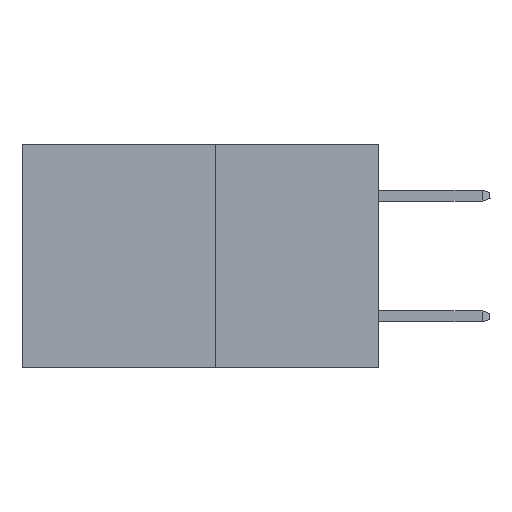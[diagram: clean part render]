
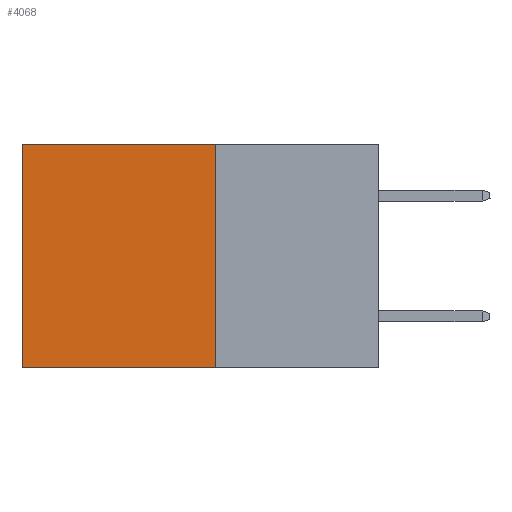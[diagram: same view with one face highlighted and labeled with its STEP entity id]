
A CAD part, left-side view. The second image highlights one B-rep face of the part: STEP entity #4068.
In plain terms, the highlighted planar face has unit normal (-1, 0, 0).
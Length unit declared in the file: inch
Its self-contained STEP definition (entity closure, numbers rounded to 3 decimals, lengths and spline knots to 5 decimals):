
#2 = EDGE_CURVE ( 'NONE', #4968, #7295, #2252, .T. ) ;
#373 = DIRECTION ( 'NONE',  ( 0., 1., 0. ) ) ;
#1313 = CARTESIAN_POINT ( 'NONE',  ( 0.277, 0.27, -0.37 ) ) ;
#2153 = CARTESIAN_POINT ( 'NONE',  ( 0.277, 0.59, -0.37 ) ) ;
#2252 = LINE ( 'NONE', #7698, #13037 ) ;
#2348 = VECTOR ( 'NONE', #8256, 39.37008 ) ;
#3199 = EDGE_CURVE ( 'NONE', #11133, #3321, #8616, .T. ) ;
#3321 = VERTEX_POINT ( 'NONE', #1313 ) ;
#3375 = AXIS2_PLACEMENT_3D ( 'NONE', #12859, #12370, #12385 ) ;
#3551 = LINE ( 'NONE', #4149, #8807 ) ;
#3883 = ORIENTED_EDGE ( 'NONE', *, *, #12152, .T. ) ;
#4068 = ADVANCED_FACE ( 'NONE', ( #10732 ), #12300, .F. ) ;
#4149 = CARTESIAN_POINT ( 'NONE',  ( 0.277, 0.27, -0.37 ) ) ;
#4968 = VERTEX_POINT ( 'NONE', #12629 ) ;
#6753 = CARTESIAN_POINT ( 'NONE',  ( 0.277, 0.27, 0. ) ) ;
#6771 = CARTESIAN_POINT ( 'NONE',  ( 0.277, 0.27, -0.37 ) ) ;
#7295 = VERTEX_POINT ( 'NONE', #2153 ) ;
#7533 = ORIENTED_EDGE ( 'NONE', *, *, #12510, .F. ) ;
#7534 = VECTOR ( 'NONE', #373, 39.37008 ) ;
#7698 = CARTESIAN_POINT ( 'NONE',  ( 0.277, 0.59, -0.37 ) ) ;
#7710 = DIRECTION ( 'NONE',  ( 0., 0., -1. ) ) ;
#7755 = EDGE_LOOP ( 'NONE', ( #8339, #7533, #13359, #3883 ) ) ;
#8256 = DIRECTION ( 'NONE',  ( 0., 0., -1. ) ) ;
#8339 = ORIENTED_EDGE ( 'NONE', *, *, #2, .T. ) ;
#8616 = LINE ( 'NONE', #6771, #2348 ) ;
#8807 = VECTOR ( 'NONE', #12500, 39.37008 ) ;
#9861 = CARTESIAN_POINT ( 'NONE',  ( 0.277, 0.27, 0. ) ) ;
#10641 = LINE ( 'NONE', #9861, #7534 ) ;
#10732 = FACE_OUTER_BOUND ( 'NONE', #7755, .T. ) ;
#11133 = VERTEX_POINT ( 'NONE', #6753 ) ;
#12152 = EDGE_CURVE ( 'NONE', #11133, #4968, #10641, .T. ) ;
#12300 = PLANE ( 'NONE',  #3375 ) ;
#12370 = DIRECTION ( 'NONE',  ( 1., 0., 0. ) ) ;
#12385 = DIRECTION ( 'NONE',  ( 0., 0., -1. ) ) ;
#12500 = DIRECTION ( 'NONE',  ( 0., 1., 0. ) ) ;
#12510 = EDGE_CURVE ( 'NONE', #3321, #7295, #3551, .T. ) ;
#12629 = CARTESIAN_POINT ( 'NONE',  ( 0.277, 0.59, 0. ) ) ;
#12859 = CARTESIAN_POINT ( 'NONE',  ( 0.277, 0.27, -0.37 ) ) ;
#13037 = VECTOR ( 'NONE', #7710, 39.37008 ) ;
#13359 = ORIENTED_EDGE ( 'NONE', *, *, #3199, .F. ) ;
